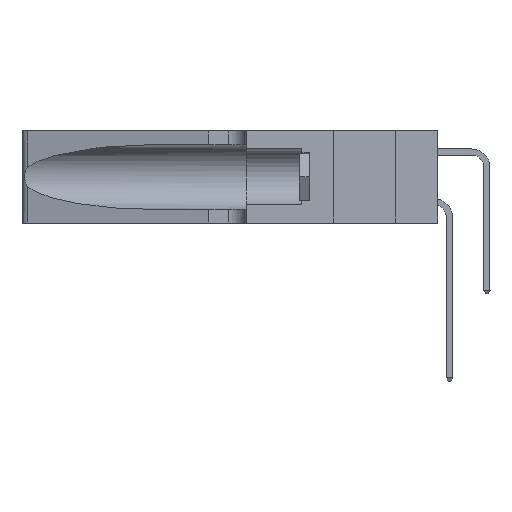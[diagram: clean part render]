
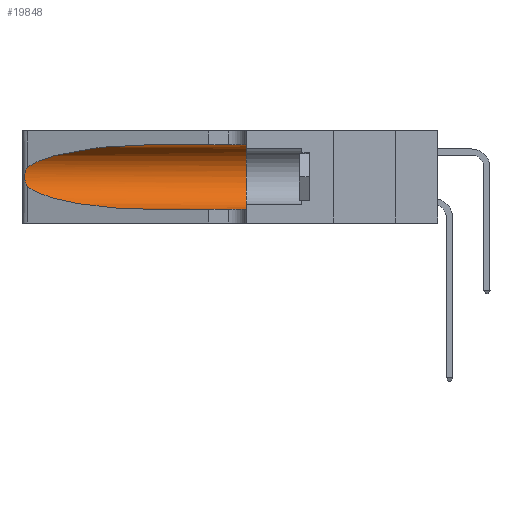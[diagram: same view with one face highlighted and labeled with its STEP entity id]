
A CAD part, left-side view. The second image highlights one B-rep face of the part: STEP entity #19848.
In plain terms, the highlighted cylindrical face has radius 3.308 mm (diameter 6.617 mm), a partial arc.
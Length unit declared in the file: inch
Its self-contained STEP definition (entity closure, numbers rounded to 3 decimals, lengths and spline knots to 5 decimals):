
#181 = ORIENTED_EDGE ( 'NONE', *, *, #2058, .T. ) ;
#294 = AXIS2_PLACEMENT_3D ( 'NONE', #28317, #9240, #12054 ) ;
#366 =( BOUNDED_CURVE ( )  B_SPLINE_CURVE ( 3, ( #27372, #30634, #29027, #15099 ),
 .UNSPECIFIED., .F., .T. ) 
 B_SPLINE_CURVE_WITH_KNOTS ( ( 4, 4 ),
 ( 3.44316, 4.71239 ),
 .UNSPECIFIED. ) 
 CURVE ( )  GEOMETRIC_REPRESENTATION_ITEM ( )  RATIONAL_B_SPLINE_CURVE ( ( 1., 0.87, 0.87, 1. ) ) 
 REPRESENTATION_ITEM ( '' )  );
#649 = EDGE_CURVE ( 'NONE', #28794, #27144, #5056, .T. ) ;
#1003 = ORIENTED_EDGE ( 'NONE', *, *, #13480, .T. ) ;
#1800 = VERTEX_POINT ( 'NONE', #31869 ) ;
#2058 = EDGE_CURVE ( 'NONE', #28815, #24610, #20733, .T. ) ;
#2093 = VECTOR ( 'NONE', #5797, 39.37008 ) ;
#2202 = CARTESIAN_POINT ( 'NONE',  ( 0.18966, 0.96281, 0.31525 ) ) ;
#2314 = CARTESIAN_POINT ( 'NONE',  ( 0.1305, 0.72297, 0.31525 ) ) ;
#3032 = DIRECTION ( 'NONE',  ( 0., -1., 0. ) ) ;
#4171 = ORIENTED_EDGE ( 'NONE', *, *, #28977, .T. ) ;
#5056 = LINE ( 'NONE', #19108, #2093 ) ;
#5768 = VERTEX_POINT ( 'NONE', #15343 ) ;
#5797 = DIRECTION ( 'NONE',  ( 0., -1., 0. ) ) ;
#6743 = CARTESIAN_POINT ( 'NONE',  ( 0.26075, 1.23896, 0.178 ) ) ;
#6878 = CARTESIAN_POINT ( 'NONE',  ( 0.25487, 1.22718, 0.22369 ) ) ;
#7119 = CARTESIAN_POINT ( 'NONE',  ( 0.25789, 1.23486, 0.15765 ) ) ;
#7172 = CARTESIAN_POINT ( 'NONE',  ( 0.2373, 1.15595, 0.28018 ) ) ;
#9181 = EDGE_LOOP ( 'NONE', ( #181, #4171, #1003, #26404, #20130, #21196 ) ) ;
#9240 = DIRECTION ( 'NONE',  ( 0., -1., 0. ) ) ;
#9481 = CARTESIAN_POINT ( 'NONE',  ( 0.25555, 1.22994, 0.2215 ) ) ;
#12054 = DIRECTION ( 'NONE',  ( 0., 0., -1. ) ) ;
#12829 = CARTESIAN_POINT ( 'NONE',  ( 0.25487, 1.22718, 0.22369 ) ) ;
#13402 = CIRCLE ( 'NONE', #29878, 0.13025 ) ;
#13480 = EDGE_CURVE ( 'NONE', #1800, #28794, #366, .T. ) ;
#13551 = EDGE_CURVE ( 'NONE', #5768, #27144, #13402, .T. ) ;
#14513 = FACE_OUTER_BOUND ( 'NONE', #9181, .T. ) ;
#14731 = CARTESIAN_POINT ( 'NONE',  ( 0.26018, 1.23835, 0.19895 ) ) ;
#15099 = CARTESIAN_POINT ( 'NONE',  ( 0.1305, 0.72297, 0.05475 ) ) ;
#15343 = CARTESIAN_POINT ( 'NONE',  ( 0.1305, 0.35, 0.31525 ) ) ;
#15586 = DIRECTION ( 'NONE',  ( 0., 1., 0. ) ) ;
#16145 = VECTOR ( 'NONE', #3032, 39.37008 ) ;
#17422 = CARTESIAN_POINT ( 'NONE',  ( 0.26017, 1.23833, 0.17102 ) ) ;
#17551 = CARTESIAN_POINT ( 'NONE',  ( 0.25555, 1.22993, 0.14849 ) ) ;
#17684 = CARTESIAN_POINT ( 'NONE',  ( 0.25854, 1.2359, 0.20912 ) ) ;
#17709 = CARTESIAN_POINT ( 'NONE',  ( 0.1305, 0.35, 0.05475 ) ) ;
#17813 = CARTESIAN_POINT ( 'NONE',  ( 0.26075, 1.23896, 0.19203 ) ) ;
#18535 = DIRECTION ( 'NONE',  ( 0., 0., 1. ) ) ;
#19108 = CARTESIAN_POINT ( 'NONE',  ( 0.1305, 1.61858, 0.05475 ) ) ;
#19160 = CYLINDRICAL_SURFACE ( 'NONE', #294, 0.13025 ) ;
#19341 = CARTESIAN_POINT ( 'NONE',  ( 0.1305, 0.72297, 0.05475 ) ) ;
#19848 = ADVANCED_FACE ( 'NONE', ( #14513 ), #19160, .F. ) ;
#20130 = ORIENTED_EDGE ( 'NONE', *, *, #13551, .F. ) ;
#20733 =( BOUNDED_CURVE ( )  B_SPLINE_CURVE ( 3, ( #2314, #2202, #7172, #25458 ),
 .UNSPECIFIED., .F., .T. ) 
 B_SPLINE_CURVE_WITH_KNOTS ( ( 4, 4 ),
 ( 1.5708, 2.84003 ),
 .UNSPECIFIED. ) 
 CURVE ( )  GEOMETRIC_REPRESENTATION_ITEM ( )  RATIONAL_B_SPLINE_CURVE ( ( 1., 0.87, 0.87, 1. ) ) 
 REPRESENTATION_ITEM ( '' )  );
#21021 = EDGE_CURVE ( 'NONE', #28815, #5768, #27518, .T. ) ;
#21196 = ORIENTED_EDGE ( 'NONE', *, *, #21021, .F. ) ;
#23241 = CARTESIAN_POINT ( 'NONE',  ( 0.25856, 1.23593, 0.16098 ) ) ;
#23991 = B_SPLINE_CURVE_WITH_KNOTS ( 'NONE', 3,
 ( #6878, #9481, #31268, #31024, #17684, #14731, #17813, #6743, #17422, #23241, #7119, #25694, #17551, #33776 ),
 .UNSPECIFIED., .F., .F.,
 ( 4, 2, 2, 2, 2, 2, 4 ),
 ( 0., 0.00027, 0.00053, 0.00107, 0.0016, 0.00187, 0.00214 ),
 .UNSPECIFIED. ) ;
#24543 = CARTESIAN_POINT ( 'NONE',  ( 0.1305, 0.72297, 0.31525 ) ) ;
#24610 = VERTEX_POINT ( 'NONE', #12829 ) ;
#25458 = CARTESIAN_POINT ( 'NONE',  ( 0.25487, 1.22718, 0.22369 ) ) ;
#25694 = CARTESIAN_POINT ( 'NONE',  ( 0.25639, 1.23186, 0.15144 ) ) ;
#26404 = ORIENTED_EDGE ( 'NONE', *, *, #649, .T. ) ;
#27144 = VERTEX_POINT ( 'NONE', #17709 ) ;
#27372 = CARTESIAN_POINT ( 'NONE',  ( 0.25487, 1.22718, 0.14631 ) ) ;
#27518 = LINE ( 'NONE', #30226, #16145 ) ;
#28317 = CARTESIAN_POINT ( 'NONE',  ( 0.1305, 1.61858, 0.185 ) ) ;
#28794 = VERTEX_POINT ( 'NONE', #19341 ) ;
#28815 = VERTEX_POINT ( 'NONE', #24543 ) ;
#28977 = EDGE_CURVE ( 'NONE', #24610, #1800, #23991, .T. ) ;
#29027 = CARTESIAN_POINT ( 'NONE',  ( 0.18966, 0.96281, 0.05475 ) ) ;
#29878 = AXIS2_PLACEMENT_3D ( 'NONE', #34852, #15586, #18535 ) ;
#30226 = CARTESIAN_POINT ( 'NONE',  ( 0.1305, 1.61858, 0.31525 ) ) ;
#30634 = CARTESIAN_POINT ( 'NONE',  ( 0.2373, 1.15595, 0.08982 ) ) ;
#31024 = CARTESIAN_POINT ( 'NONE',  ( 0.25787, 1.23484, 0.2124 ) ) ;
#31268 = CARTESIAN_POINT ( 'NONE',  ( 0.25639, 1.23184, 0.21858 ) ) ;
#31869 = CARTESIAN_POINT ( 'NONE',  ( 0.25487, 1.22718, 0.14631 ) ) ;
#33776 = CARTESIAN_POINT ( 'NONE',  ( 0.25487, 1.22718, 0.14631 ) ) ;
#34852 = CARTESIAN_POINT ( 'NONE',  ( 0.1305, 0.35, 0.185 ) ) ;
